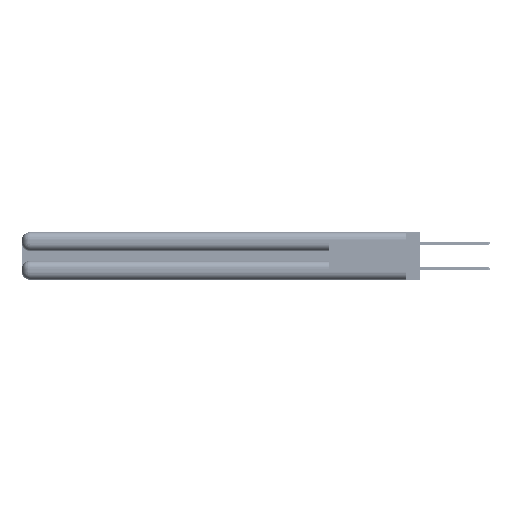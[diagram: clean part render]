
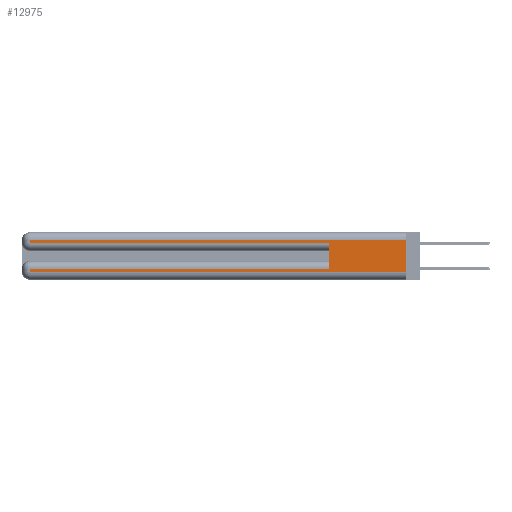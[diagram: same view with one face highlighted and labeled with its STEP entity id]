
A CAD part, left-side view. The second image highlights one B-rep face of the part: STEP entity #12975.
In plain terms, the highlighted planar face has unit normal (-1, 0, 0).
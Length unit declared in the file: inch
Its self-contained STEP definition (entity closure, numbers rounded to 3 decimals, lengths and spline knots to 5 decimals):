
#768 = DIRECTION ( 'NONE',  ( 0., -1., 0. ) ) ;
#5280 = ORIENTED_EDGE ( 'NONE', *, *, #41083, .F. ) ;
#6015 = EDGE_CURVE ( 'NONE', #11860, #52609, #26810, .T. ) ;
#7472 = CARTESIAN_POINT ( 'NONE',  ( 0., 0., 0.37 ) ) ;
#7964 = VECTOR ( 'NONE', #49579, 39.37008 ) ;
#9112 = LINE ( 'NONE', #16699, #42929 ) ;
#9246 = ORIENTED_EDGE ( 'NONE', *, *, #55523, .T. ) ;
#9382 = VERTEX_POINT ( 'NONE', #41998 ) ;
#9962 = DIRECTION ( 'NONE',  ( 0., 0., 1. ) ) ;
#11325 = LINE ( 'NONE', #28672, #56880 ) ;
#11860 = VERTEX_POINT ( 'NONE', #35964 ) ;
#12611 = EDGE_CURVE ( 'NONE', #22670, #46188, #23168, .T. ) ;
#12961 = VERTEX_POINT ( 'NONE', #25082 ) ;
#12975 = ADVANCED_FACE ( 'NONE', ( #34809 ), #38349, .F. ) ;
#14636 = VERTEX_POINT ( 'NONE', #22486 ) ;
#16699 = CARTESIAN_POINT ( 'NONE',  ( 0., 0., 0.31 ) ) ;
#18899 = ORIENTED_EDGE ( 'NONE', *, *, #43610, .T. ) ;
#19171 = CARTESIAN_POINT ( 'NONE',  ( 0., 0.6, 0.085 ) ) ;
#19557 = CARTESIAN_POINT ( 'NONE',  ( 0., 0., 0.37 ) ) ;
#20100 = EDGE_CURVE ( 'NONE', #12961, #22670, #43205, .T. ) ;
#21135 = ORIENTED_EDGE ( 'NONE', *, *, #20100, .T. ) ;
#21666 = VECTOR ( 'NONE', #51088, 39.37008 ) ;
#22435 = LINE ( 'NONE', #33433, #44443 ) ;
#22486 = CARTESIAN_POINT ( 'NONE',  ( 0., 2.94, 0.06 ) ) ;
#22670 = VERTEX_POINT ( 'NONE', #40473 ) ;
#23086 = EDGE_CURVE ( 'NONE', #11860, #12961, #9112, .T. ) ;
#23168 = LINE ( 'NONE', #40349, #42423 ) ;
#25082 = CARTESIAN_POINT ( 'NONE',  ( 0., 2.94, 0.31 ) ) ;
#25390 = VECTOR ( 'NONE', #9962, 39.37008 ) ;
#26810 = LINE ( 'NONE', #19557, #50234 ) ;
#28672 = CARTESIAN_POINT ( 'NONE',  ( 0., 0., 0.085 ) ) ;
#29535 = AXIS2_PLACEMENT_3D ( 'NONE', #7472, #56116, #29707 ) ;
#29707 = DIRECTION ( 'NONE',  ( 0., 0., -1. ) ) ;
#30894 = VERTEX_POINT ( 'NONE', #19171 ) ;
#33122 = DIRECTION ( 'NONE',  ( 0., 1., 0. ) ) ;
#33433 = CARTESIAN_POINT ( 'NONE',  ( 0., 2.94, 0.37 ) ) ;
#33440 = CARTESIAN_POINT ( 'NONE',  ( 0., 0., 0.06 ) ) ;
#34809 = FACE_OUTER_BOUND ( 'NONE', #45878, .T. ) ;
#35155 = CARTESIAN_POINT ( 'NONE',  ( 0., 0.6, 0.285 ) ) ;
#35964 = CARTESIAN_POINT ( 'NONE',  ( 0., 0., 0.31 ) ) ;
#36406 = CARTESIAN_POINT ( 'NONE',  ( 0., 0.6, 0.145 ) ) ;
#37842 = DIRECTION ( 'NONE',  ( 0., 0., -1. ) ) ;
#38349 = PLANE ( 'NONE',  #29535 ) ;
#38689 = ORIENTED_EDGE ( 'NONE', *, *, #12611, .T. ) ;
#40349 = CARTESIAN_POINT ( 'NONE',  ( 0., 0., 0.285 ) ) ;
#40473 = CARTESIAN_POINT ( 'NONE',  ( 0., 2.94, 0.285 ) ) ;
#41083 = EDGE_CURVE ( 'NONE', #30894, #46188, #47419, .T. ) ;
#41479 = DIRECTION ( 'NONE',  ( 0., 0., -1. ) ) ;
#41998 = CARTESIAN_POINT ( 'NONE',  ( 0., 2.94, 0.085 ) ) ;
#42423 = VECTOR ( 'NONE', #768, 39.37008 ) ;
#42929 = VECTOR ( 'NONE', #47516, 39.37008 ) ;
#43205 = LINE ( 'NONE', #45136, #7964 ) ;
#43610 = EDGE_CURVE ( 'NONE', #9382, #14636, #22435, .T. ) ;
#43619 = ORIENTED_EDGE ( 'NONE', *, *, #6015, .F. ) ;
#44272 = EDGE_CURVE ( 'NONE', #14636, #52609, #46438, .T. ) ;
#44443 = VECTOR ( 'NONE', #37842, 39.37008 ) ;
#45136 = CARTESIAN_POINT ( 'NONE',  ( 0., 2.94, 0.37 ) ) ;
#45878 = EDGE_LOOP ( 'NONE', ( #43619, #55796, #21135, #38689, #5280, #9246, #18899, #53257 ) ) ;
#46188 = VERTEX_POINT ( 'NONE', #35155 ) ;
#46438 = LINE ( 'NONE', #50903, #21666 ) ;
#47419 = LINE ( 'NONE', #36406, #25390 ) ;
#47516 = DIRECTION ( 'NONE',  ( 0., 1., 0. ) ) ;
#49579 = DIRECTION ( 'NONE',  ( 0., 0., -1. ) ) ;
#50234 = VECTOR ( 'NONE', #41479, 39.37008 ) ;
#50903 = CARTESIAN_POINT ( 'NONE',  ( 0., 0., 0.06 ) ) ;
#51088 = DIRECTION ( 'NONE',  ( 0., -1., 0. ) ) ;
#52609 = VERTEX_POINT ( 'NONE', #33440 ) ;
#53257 = ORIENTED_EDGE ( 'NONE', *, *, #44272, .T. ) ;
#55523 = EDGE_CURVE ( 'NONE', #30894, #9382, #11325, .T. ) ;
#55796 = ORIENTED_EDGE ( 'NONE', *, *, #23086, .T. ) ;
#56116 = DIRECTION ( 'NONE',  ( 1., 0., 0. ) ) ;
#56880 = VECTOR ( 'NONE', #33122, 39.37008 ) ;
